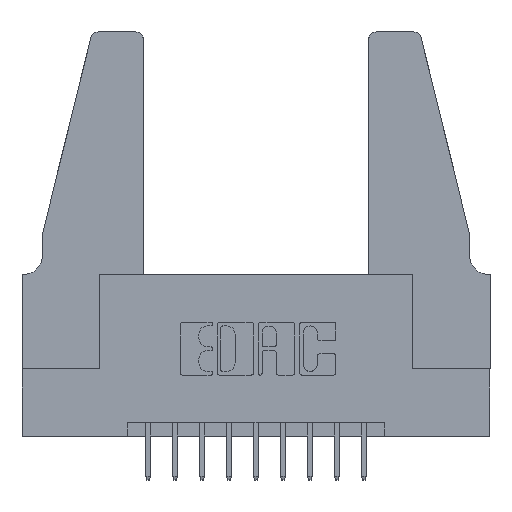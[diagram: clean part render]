
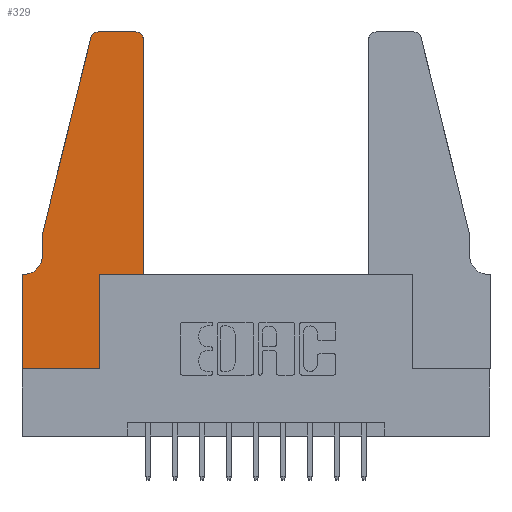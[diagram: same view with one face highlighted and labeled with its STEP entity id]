
A CAD part, top view. The second image highlights one B-rep face of the part: STEP entity #329.
In plain terms, the highlighted planar face has unit normal (0, 0, 1).
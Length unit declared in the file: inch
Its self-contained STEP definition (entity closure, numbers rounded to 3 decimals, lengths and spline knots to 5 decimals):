
#24 = VECTOR ( 'NONE', #9649, 39.37008 ) ;
#151 = LINE ( 'NONE', #10203, #8938 ) ;
#329 = ADVANCED_FACE ( 'NONE', ( #13467 ), #2738, .T. ) ;
#340 = CARTESIAN_POINT ( 'NONE',  ( 0.2865, 0.35, 0.37 ) ) ;
#451 = EDGE_CURVE ( 'NONE', #9761, #11652, #8477, .T. ) ;
#517 = CARTESIAN_POINT ( 'NONE',  ( 0.4505, 1.22, 0.37 ) ) ;
#724 = ORIENTED_EDGE ( 'NONE', *, *, #6743, .T. ) ;
#910 = CARTESIAN_POINT ( 'NONE',  ( 0.2865, 0., 0.37 ) ) ;
#1133 = LINE ( 'NONE', #1801, #11070 ) ;
#1258 = EDGE_CURVE ( 'NONE', #10676, #2866, #151, .T. ) ;
#1434 = VERTEX_POINT ( 'NONE', #910 ) ;
#1452 = DIRECTION ( 'NONE',  ( 1., 0., 0. ) ) ;
#1575 = CARTESIAN_POINT ( 'NONE',  ( 0., 0.35, 0.37 ) ) ;
#1751 = DIRECTION ( 'NONE',  ( 0., 1., 0. ) ) ;
#1801 = CARTESIAN_POINT ( 'NONE',  ( 0.4505, 0.35, 0.37 ) ) ;
#1972 = CARTESIAN_POINT ( 'NONE',  ( 0.0755, 0.35, 0.37 ) ) ;
#2118 = ORIENTED_EDGE ( 'NONE', *, *, #4604, .T. ) ;
#2183 = ORIENTED_EDGE ( 'NONE', *, *, #2727, .T. ) ;
#2256 = LINE ( 'NONE', #10535, #6707 ) ;
#2311 = DIRECTION ( 'NONE',  ( 0., -1., 0. ) ) ;
#2727 = EDGE_CURVE ( 'NONE', #5582, #9761, #1133, .T. ) ;
#2729 = CARTESIAN_POINT ( 'NONE',  ( 0.0755, 0.5, 0.37 ) ) ;
#2738 = PLANE ( 'NONE',  #3429 ) ;
#2845 = DIRECTION ( 'NONE',  ( 0., 1., 0. ) ) ;
#2866 = VERTEX_POINT ( 'NONE', #2729 ) ;
#3166 = ORIENTED_EDGE ( 'NONE', *, *, #8137, .T. ) ;
#3300 = AXIS2_PLACEMENT_3D ( 'NONE', #13249, #9010, #6817 ) ;
#3429 = AXIS2_PLACEMENT_3D ( 'NONE', #1575, #10159, #13312 ) ;
#3636 = CARTESIAN_POINT ( 'NONE',  ( 0., 0., 0.37 ) ) ;
#3862 = VERTEX_POINT ( 'NONE', #5008 ) ;
#4434 = ORIENTED_EDGE ( 'NONE', *, *, #1258, .T. ) ;
#4604 = EDGE_CURVE ( 'NONE', #3862, #1434, #12831, .T. ) ;
#4794 = AXIS2_PLACEMENT_3D ( 'NONE', #6067, #7211, #8186 ) ;
#4813 = DIRECTION ( 'NONE',  ( 0., 0., 1. ) ) ;
#4818 = CIRCLE ( 'NONE', #8960, 0.03 ) ;
#4845 = CARTESIAN_POINT ( 'NONE',  ( 0.4505, 0.35, 0.37 ) ) ;
#5008 = CARTESIAN_POINT ( 'NONE',  ( 0., 0., 0.37 ) ) ;
#5310 = VECTOR ( 'NONE', #1751, 39.37008 ) ;
#5371 = EDGE_CURVE ( 'NONE', #6080, #9694, #8810, .T. ) ;
#5392 = EDGE_CURVE ( 'NONE', #2866, #9321, #5652, .T. ) ;
#5400 = VECTOR ( 'NONE', #2845, 39.37008 ) ;
#5582 = VERTEX_POINT ( 'NONE', #340 ) ;
#5652 = LINE ( 'NONE', #10459, #10825 ) ;
#5688 = EDGE_CURVE ( 'NONE', #11652, #6481, #4818, .T. ) ;
#5714 = VECTOR ( 'NONE', #9304, 39.37008 ) ;
#5851 = ORIENTED_EDGE ( 'NONE', *, *, #8698, .T. ) ;
#6067 = CARTESIAN_POINT ( 'NONE',  ( 0.0055, 0.42, 0.37 ) ) ;
#6080 = VERTEX_POINT ( 'NONE', #6086 ) ;
#6086 = CARTESIAN_POINT ( 'NONE',  ( 0.0055, 0.35, 0.37 ) ) ;
#6114 = CIRCLE ( 'NONE', #4794, 0.07 ) ;
#6149 = CARTESIAN_POINT ( 'NONE',  ( 0.25487, 1.22718, 0.37 ) ) ;
#6201 = CARTESIAN_POINT ( 'NONE',  ( 0.284, 1.25, 0.37 ) ) ;
#6318 = CARTESIAN_POINT ( 'NONE',  ( 0.2605, 1.25, 0.37 ) ) ;
#6481 = VERTEX_POINT ( 'NONE', #10199 ) ;
#6707 = VECTOR ( 'NONE', #9540, 39.37008 ) ;
#6743 = EDGE_CURVE ( 'NONE', #9321, #6080, #6114, .T. ) ;
#6776 = ORIENTED_EDGE ( 'NONE', *, *, #5688, .T. ) ;
#6817 = DIRECTION ( 'NONE',  ( 1., 0., 0. ) ) ;
#6829 = VERTEX_POINT ( 'NONE', #6201 ) ;
#7017 = DIRECTION ( 'NONE',  ( -0.239, -0.971, 0. ) ) ;
#7211 = DIRECTION ( 'NONE',  ( 0., 0., -1. ) ) ;
#7526 = CARTESIAN_POINT ( 'NONE',  ( 0.4505, 0.35, 0.37 ) ) ;
#7572 = EDGE_CURVE ( 'NONE', #6829, #10676, #8586, .T. ) ;
#8137 = EDGE_CURVE ( 'NONE', #1434, #5582, #8397, .T. ) ;
#8186 = DIRECTION ( 'NONE',  ( -1., 0., 0. ) ) ;
#8196 = LINE ( 'NONE', #6318, #5714 ) ;
#8321 = EDGE_LOOP ( 'NONE', ( #5851, #10630, #4434, #12362, #724, #13663, #10801, #2118, #3166, #2183, #12255, #6776 ) ) ;
#8397 = LINE ( 'NONE', #11348, #5400 ) ;
#8477 = LINE ( 'NONE', #7526, #5310 ) ;
#8586 = CIRCLE ( 'NONE', #3300, 0.03 ) ;
#8698 = EDGE_CURVE ( 'NONE', #6481, #6829, #8196, .T. ) ;
#8810 = LINE ( 'NONE', #1972, #24 ) ;
#8938 = VECTOR ( 'NONE', #7017, 39.37008 ) ;
#8960 = AXIS2_PLACEMENT_3D ( 'NONE', #10162, #4813, #12283 ) ;
#9010 = DIRECTION ( 'NONE',  ( 0., 0., 1. ) ) ;
#9304 = DIRECTION ( 'NONE',  ( -1., 0., 0. ) ) ;
#9321 = VERTEX_POINT ( 'NONE', #10488 ) ;
#9540 = DIRECTION ( 'NONE',  ( 0., -1., 0. ) ) ;
#9649 = DIRECTION ( 'NONE',  ( -1., 0., 0. ) ) ;
#9694 = VERTEX_POINT ( 'NONE', #12903 ) ;
#9761 = VERTEX_POINT ( 'NONE', #4845 ) ;
#10159 = DIRECTION ( 'NONE',  ( 0., 0., 1. ) ) ;
#10162 = CARTESIAN_POINT ( 'NONE',  ( 0.4205, 1.22, 0.37 ) ) ;
#10199 = CARTESIAN_POINT ( 'NONE',  ( 0.4205, 1.25, 0.37 ) ) ;
#10203 = CARTESIAN_POINT ( 'NONE',  ( 0.0755, 0.5, 0.37 ) ) ;
#10459 = CARTESIAN_POINT ( 'NONE',  ( 0.0755, 0.5, 0.37 ) ) ;
#10488 = CARTESIAN_POINT ( 'NONE',  ( 0.0755, 0.42, 0.37 ) ) ;
#10535 = CARTESIAN_POINT ( 'NONE',  ( 0., 0., 0.37 ) ) ;
#10630 = ORIENTED_EDGE ( 'NONE', *, *, #7572, .T. ) ;
#10676 = VERTEX_POINT ( 'NONE', #6149 ) ;
#10801 = ORIENTED_EDGE ( 'NONE', *, *, #12363, .T. ) ;
#10825 = VECTOR ( 'NONE', #2311, 39.37008 ) ;
#11070 = VECTOR ( 'NONE', #13571, 39.37008 ) ;
#11326 = VECTOR ( 'NONE', #1452, 39.37008 ) ;
#11348 = CARTESIAN_POINT ( 'NONE',  ( 0.2865, 0.35, 0.37 ) ) ;
#11652 = VERTEX_POINT ( 'NONE', #517 ) ;
#12255 = ORIENTED_EDGE ( 'NONE', *, *, #451, .T. ) ;
#12283 = DIRECTION ( 'NONE',  ( 1., 0., 0. ) ) ;
#12362 = ORIENTED_EDGE ( 'NONE', *, *, #5392, .T. ) ;
#12363 = EDGE_CURVE ( 'NONE', #9694, #3862, #2256, .T. ) ;
#12831 = LINE ( 'NONE', #3636, #11326 ) ;
#12903 = CARTESIAN_POINT ( 'NONE',  ( 0., 0.35, 0.37 ) ) ;
#13249 = CARTESIAN_POINT ( 'NONE',  ( 0.284, 1.22, 0.37 ) ) ;
#13312 = DIRECTION ( 'NONE',  ( 1., 0., 0. ) ) ;
#13467 = FACE_OUTER_BOUND ( 'NONE', #8321, .T. ) ;
#13571 = DIRECTION ( 'NONE',  ( 1., 0., 0. ) ) ;
#13663 = ORIENTED_EDGE ( 'NONE', *, *, #5371, .T. ) ;
